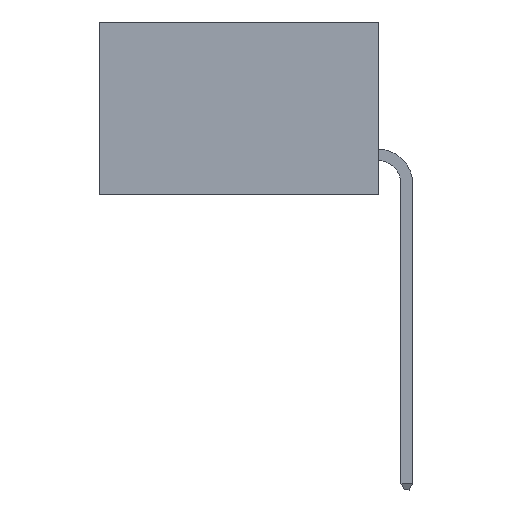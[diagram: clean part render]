
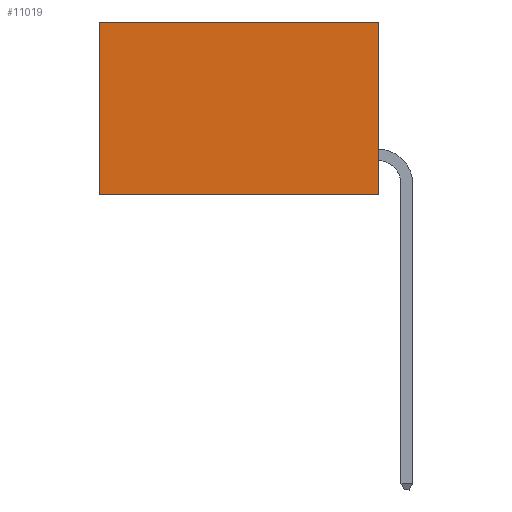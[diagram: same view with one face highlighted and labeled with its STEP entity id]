
A CAD part, left-side view. The second image highlights one B-rep face of the part: STEP entity #11019.
In plain terms, the highlighted planar face has unit normal (-1, 0, 0).
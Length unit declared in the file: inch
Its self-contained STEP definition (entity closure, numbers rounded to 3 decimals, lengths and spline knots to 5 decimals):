
#351 = CARTESIAN_POINT ( 'NONE',  ( 0.298, 0., 0. ) ) ;
#435 = VECTOR ( 'NONE', #5916, 39.37008 ) ;
#581 = DIRECTION ( 'NONE',  ( 1., 0., 0. ) ) ;
#1634 = VECTOR ( 'NONE', #4852, 39.37008 ) ;
#1665 = LINE ( 'NONE', #3736, #13345 ) ;
#2264 = DIRECTION ( 'NONE',  ( 0., 1., 0. ) ) ;
#2553 = VERTEX_POINT ( 'NONE', #12331 ) ;
#3329 = LINE ( 'NONE', #13603, #435 ) ;
#3736 = CARTESIAN_POINT ( 'NONE',  ( 0.298, 0., 0. ) ) ;
#4185 = EDGE_CURVE ( 'NONE', #13165, #10245, #1665, .T. ) ;
#4221 = EDGE_LOOP ( 'NONE', ( #4894, #12606, #7073, #4723 ) ) ;
#4723 = ORIENTED_EDGE ( 'NONE', *, *, #7892, .T. ) ;
#4812 = LINE ( 'NONE', #351, #1634 ) ;
#4852 = DIRECTION ( 'NONE',  ( 0., 1., 0. ) ) ;
#4894 = ORIENTED_EDGE ( 'NONE', *, *, #7762, .T. ) ;
#5835 = VERTEX_POINT ( 'NONE', #9296 ) ;
#5916 = DIRECTION ( 'NONE',  ( 0., 0., -1. ) ) ;
#7073 = ORIENTED_EDGE ( 'NONE', *, *, #4185, .F. ) ;
#7150 = LINE ( 'NONE', #8729, #12811 ) ;
#7181 = FACE_OUTER_BOUND ( 'NONE', #4221, .T. ) ;
#7339 = CARTESIAN_POINT ( 'NONE',  ( 0.298, 0., 0. ) ) ;
#7762 = EDGE_CURVE ( 'NONE', #2553, #5835, #3329, .T. ) ;
#7892 = EDGE_CURVE ( 'NONE', #13165, #2553, #4812, .T. ) ;
#8073 = AXIS2_PLACEMENT_3D ( 'NONE', #12359, #581, #8104 ) ;
#8104 = DIRECTION ( 'NONE',  ( 0., 0., -1. ) ) ;
#8729 = CARTESIAN_POINT ( 'NONE',  ( 0.298, 0., -0.37 ) ) ;
#9296 = CARTESIAN_POINT ( 'NONE',  ( 0.298, 0.6, -0.37 ) ) ;
#10245 = VERTEX_POINT ( 'NONE', #12146 ) ;
#11019 = ADVANCED_FACE ( 'NONE', ( #7181 ), #13384, .F. ) ;
#11826 = EDGE_CURVE ( 'NONE', #10245, #5835, #7150, .T. ) ;
#12146 = CARTESIAN_POINT ( 'NONE',  ( 0.298, 0., -0.37 ) ) ;
#12331 = CARTESIAN_POINT ( 'NONE',  ( 0.298, 0.6, 0. ) ) ;
#12359 = CARTESIAN_POINT ( 'NONE',  ( 0.298, 0., 0. ) ) ;
#12606 = ORIENTED_EDGE ( 'NONE', *, *, #11826, .F. ) ;
#12811 = VECTOR ( 'NONE', #2264, 39.37008 ) ;
#13165 = VERTEX_POINT ( 'NONE', #7339 ) ;
#13206 = DIRECTION ( 'NONE',  ( 0., 0., -1. ) ) ;
#13345 = VECTOR ( 'NONE', #13206, 39.37008 ) ;
#13384 = PLANE ( 'NONE',  #8073 ) ;
#13603 = CARTESIAN_POINT ( 'NONE',  ( 0.298, 0.6, 0. ) ) ;
